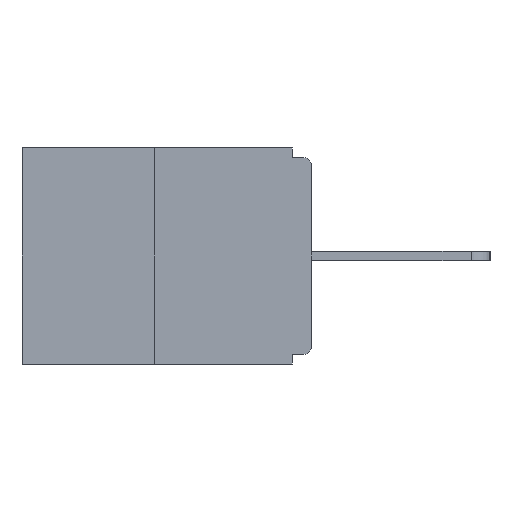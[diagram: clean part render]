
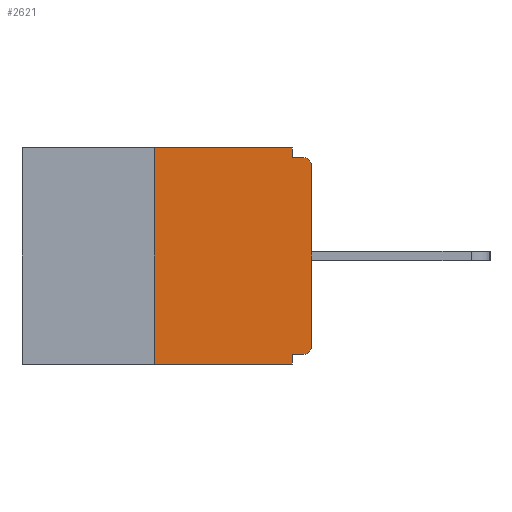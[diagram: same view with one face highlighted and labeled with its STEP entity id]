
A CAD part, left-side view. The second image highlights one B-rep face of the part: STEP entity #2621.
In plain terms, the highlighted planar face has unit normal (-1, 0, 0).
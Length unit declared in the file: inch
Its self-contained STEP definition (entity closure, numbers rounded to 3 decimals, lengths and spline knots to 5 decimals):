
#52 = EDGE_CURVE ( 'NONE', #517, #4640, #15022, .T. ) ;
#87 = DIRECTION ( 'NONE',  ( -1., 0., 0. ) ) ;
#135 = DIRECTION ( 'NONE',  ( -1., 0., 0. ) ) ;
#303 = EDGE_CURVE ( 'NONE', #4640, #12006, #5684, .T. ) ;
#331 = LINE ( 'NONE', #20862, #14048 ) ;
#517 = VERTEX_POINT ( 'NONE', #20649 ) ;
#550 = EDGE_CURVE ( 'NONE', #7376, #2566, #8849, .T. ) ;
#674 = ORIENTED_EDGE ( 'NONE', *, *, #10026, .T. ) ;
#1385 = DIRECTION ( 'NONE',  ( 0., 0., 1. ) ) ;
#1428 = EDGE_CURVE ( 'NONE', #3148, #1845, #5994, .T. ) ;
#1845 = VERTEX_POINT ( 'NONE', #5128 ) ;
#2566 = VERTEX_POINT ( 'NONE', #18493 ) ;
#2621 = ADVANCED_FACE ( 'NONE', ( #15565 ), #19017, .F. ) ;
#2706 = LINE ( 'NONE', #14358, #20209 ) ;
#3148 = VERTEX_POINT ( 'NONE', #12099 ) ;
#3382 = ORIENTED_EDGE ( 'NONE', *, *, #303, .F. ) ;
#3404 = EDGE_CURVE ( 'NONE', #7376, #12255, #7697, .T. ) ;
#3675 = EDGE_CURVE ( 'NONE', #12255, #7769, #331, .T. ) ;
#4095 = CARTESIAN_POINT ( 'NONE',  ( 0., 0.031, -0.343 ) ) ;
#4102 = CARTESIAN_POINT ( 'NONE',  ( 0., 0.46, 0. ) ) ;
#4346 = DIRECTION ( 'NONE',  ( 0., 1., 0. ) ) ;
#4487 = ORIENTED_EDGE ( 'NONE', *, *, #1428, .T. ) ;
#4640 = VERTEX_POINT ( 'NONE', #17975 ) ;
#4847 = EDGE_LOOP ( 'NONE', ( #3382, #7167, #674, #11922, #19298, #18824, #20134, #4487, #9505, #16614 ) ) ;
#5063 = DIRECTION ( 'NONE',  ( 0., 0., -1. ) ) ;
#5128 = CARTESIAN_POINT ( 'NONE',  ( 0., 0.015, -0.015 ) ) ;
#5547 = DIRECTION ( 'NONE',  ( 0., 0., -1. ) ) ;
#5637 = AXIS2_PLACEMENT_3D ( 'NONE', #15498, #87, #13717 ) ;
#5655 = CARTESIAN_POINT ( 'NONE',  ( 0., 0.031, 0. ) ) ;
#5684 = LINE ( 'NONE', #4102, #18836 ) ;
#5820 = VECTOR ( 'NONE', #4346, 39.37008 ) ;
#5994 = CIRCLE ( 'NONE', #6347, 0.015 ) ;
#6347 = AXIS2_PLACEMENT_3D ( 'NONE', #6625, #135, #11663 ) ;
#6625 = CARTESIAN_POINT ( 'NONE',  ( 0., 0.015, -0.03 ) ) ;
#7167 = ORIENTED_EDGE ( 'NONE', *, *, #52, .F. ) ;
#7376 = VERTEX_POINT ( 'NONE', #17800 ) ;
#7613 = AXIS2_PLACEMENT_3D ( 'NONE', #17026, #8543, #5063 ) ;
#7697 = LINE ( 'NONE', #11165, #5820 ) ;
#7769 = VERTEX_POINT ( 'NONE', #4095 ) ;
#8543 = DIRECTION ( 'NONE',  ( 1., 0., 0. ) ) ;
#8849 = CIRCLE ( 'NONE', #5637, 0.015 ) ;
#9505 = ORIENTED_EDGE ( 'NONE', *, *, #21201, .F. ) ;
#9545 = DIRECTION ( 'NONE',  ( 0., -1., 0. ) ) ;
#9924 = VECTOR ( 'NONE', #20492, 39.37008 ) ;
#10026 = EDGE_CURVE ( 'NONE', #517, #7769, #18818, .T. ) ;
#10662 = CARTESIAN_POINT ( 'NONE',  ( 0., 0.46, -0.343 ) ) ;
#10922 = DIRECTION ( 'NONE',  ( 0., -1., 0. ) ) ;
#11165 = CARTESIAN_POINT ( 'NONE',  ( 0., 0., -0.328 ) ) ;
#11500 = EDGE_CURVE ( 'NONE', #12006, #14013, #14151, .T. ) ;
#11663 = DIRECTION ( 'NONE',  ( 0., 0., -1. ) ) ;
#11815 = LINE ( 'NONE', #17049, #19584 ) ;
#11922 = ORIENTED_EDGE ( 'NONE', *, *, #3675, .F. ) ;
#12006 = VERTEX_POINT ( 'NONE', #18315 ) ;
#12099 = CARTESIAN_POINT ( 'NONE',  ( 0., 0., -0.03 ) ) ;
#12255 = VERTEX_POINT ( 'NONE', #14406 ) ;
#12498 = CARTESIAN_POINT ( 'NONE',  ( 0., 0.031, -0.015 ) ) ;
#13717 = DIRECTION ( 'NONE',  ( 0., 0., -1. ) ) ;
#13962 = CARTESIAN_POINT ( 'NONE',  ( 0., 0.25, 0. ) ) ;
#14013 = VERTEX_POINT ( 'NONE', #12498 ) ;
#14048 = VECTOR ( 'NONE', #5547, 39.37008 ) ;
#14151 = LINE ( 'NONE', #5655, #20602 ) ;
#14358 = CARTESIAN_POINT ( 'NONE',  ( 0., 0., -0.015 ) ) ;
#14406 = CARTESIAN_POINT ( 'NONE',  ( 0., 0.031, -0.328 ) ) ;
#15022 = LINE ( 'NONE', #13962, #18469 ) ;
#15498 = CARTESIAN_POINT ( 'NONE',  ( 0., 0.015, -0.313 ) ) ;
#15565 = FACE_OUTER_BOUND ( 'NONE', #4847, .T. ) ;
#16559 = DIRECTION ( 'NONE',  ( 0., 0., -1. ) ) ;
#16614 = ORIENTED_EDGE ( 'NONE', *, *, #11500, .F. ) ;
#17026 = CARTESIAN_POINT ( 'NONE',  ( 0., 0.46, 0. ) ) ;
#17049 = CARTESIAN_POINT ( 'NONE',  ( 0., 0., 0. ) ) ;
#17800 = CARTESIAN_POINT ( 'NONE',  ( 0., 0.015, -0.328 ) ) ;
#17975 = CARTESIAN_POINT ( 'NONE',  ( 0., 0.25, 0. ) ) ;
#18315 = CARTESIAN_POINT ( 'NONE',  ( 0., 0.031, 0. ) ) ;
#18378 = DIRECTION ( 'NONE',  ( 0., 0., 1. ) ) ;
#18469 = VECTOR ( 'NONE', #1385, 39.37008 ) ;
#18493 = CARTESIAN_POINT ( 'NONE',  ( 0., 0., -0.313 ) ) ;
#18818 = LINE ( 'NONE', #10662, #9924 ) ;
#18824 = ORIENTED_EDGE ( 'NONE', *, *, #550, .T. ) ;
#18836 = VECTOR ( 'NONE', #10922, 39.37008 ) ;
#19017 = PLANE ( 'NONE',  #7613 ) ;
#19298 = ORIENTED_EDGE ( 'NONE', *, *, #3404, .F. ) ;
#19531 = EDGE_CURVE ( 'NONE', #2566, #3148, #11815, .T. ) ;
#19584 = VECTOR ( 'NONE', #18378, 39.37008 ) ;
#20134 = ORIENTED_EDGE ( 'NONE', *, *, #19531, .T. ) ;
#20209 = VECTOR ( 'NONE', #9545, 39.37008 ) ;
#20492 = DIRECTION ( 'NONE',  ( 0., -1., 0. ) ) ;
#20602 = VECTOR ( 'NONE', #16559, 39.37008 ) ;
#20649 = CARTESIAN_POINT ( 'NONE',  ( 0., 0.25, -0.343 ) ) ;
#20862 = CARTESIAN_POINT ( 'NONE',  ( 0., 0.031, -0.343 ) ) ;
#21201 = EDGE_CURVE ( 'NONE', #14013, #1845, #2706, .T. ) ;
